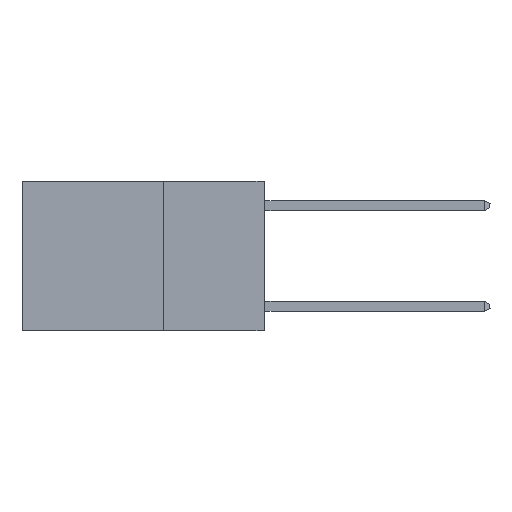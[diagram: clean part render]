
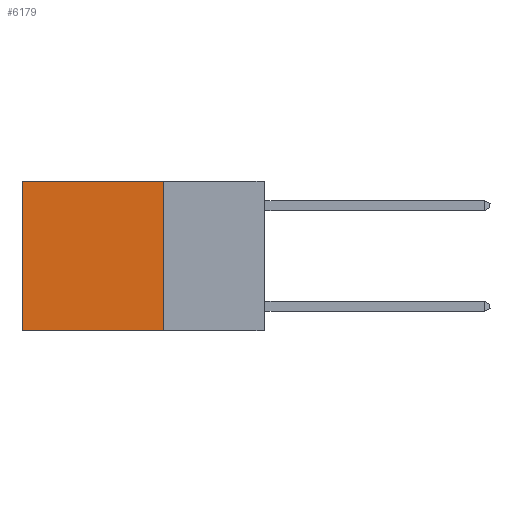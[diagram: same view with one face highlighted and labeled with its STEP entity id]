
A CAD part, left-side view. The second image highlights one B-rep face of the part: STEP entity #6179.
In plain terms, the highlighted planar face has unit normal (-1, 0, 0).
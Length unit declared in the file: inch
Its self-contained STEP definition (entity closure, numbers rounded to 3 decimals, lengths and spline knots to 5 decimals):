
#463 = VECTOR ( 'NONE', #7696, 39.37008 ) ;
#604 = DIRECTION ( 'NONE',  ( 0., 1., 0. ) ) ;
#834 = VECTOR ( 'NONE', #1040, 39.37008 ) ;
#1011 = EDGE_CURVE ( 'NONE', #14255, #8919, #1939, .T. ) ;
#1040 = DIRECTION ( 'NONE',  ( 0., 0., -1. ) ) ;
#1117 = CARTESIAN_POINT ( 'NONE',  ( 0.2625, 0.6, 0. ) ) ;
#1312 = VECTOR ( 'NONE', #604, 39.37008 ) ;
#1901 = LINE ( 'NONE', #1994, #1312 ) ;
#1939 = LINE ( 'NONE', #13079, #463 ) ;
#1994 = CARTESIAN_POINT ( 'NONE',  ( 0.2625, 0.25, -0.37 ) ) ;
#2526 = AXIS2_PLACEMENT_3D ( 'NONE', #12234, #15395, #13713 ) ;
#2606 = EDGE_CURVE ( 'NONE', #8919, #3448, #11747, .T. ) ;
#3366 = CARTESIAN_POINT ( 'NONE',  ( 0.2625, 0.25, -0.37 ) ) ;
#3448 = VERTEX_POINT ( 'NONE', #7010 ) ;
#3932 = CARTESIAN_POINT ( 'NONE',  ( 0.2625, 0.25, 0. ) ) ;
#5581 = ORIENTED_EDGE ( 'NONE', *, *, #1011, .T. ) ;
#6179 = ADVANCED_FACE ( 'NONE', ( #6669 ), #9768, .F. ) ;
#6669 = FACE_OUTER_BOUND ( 'NONE', #12794, .T. ) ;
#7010 = CARTESIAN_POINT ( 'NONE',  ( 0.2625, 0.6, -0.37 ) ) ;
#7696 = DIRECTION ( 'NONE',  ( 0., 1., 0. ) ) ;
#7801 = VECTOR ( 'NONE', #17135, 39.37008 ) ;
#8002 = LINE ( 'NONE', #9363, #834 ) ;
#8328 = EDGE_CURVE ( 'NONE', #10433, #3448, #1901, .T. ) ;
#8767 = CARTESIAN_POINT ( 'NONE',  ( 0.2625, 0.6, 0. ) ) ;
#8919 = VERTEX_POINT ( 'NONE', #1117 ) ;
#9363 = CARTESIAN_POINT ( 'NONE',  ( 0.2625, 0.25, 0. ) ) ;
#9768 = PLANE ( 'NONE',  #2526 ) ;
#9933 = ORIENTED_EDGE ( 'NONE', *, *, #13652, .F. ) ;
#10433 = VERTEX_POINT ( 'NONE', #3366 ) ;
#11747 = LINE ( 'NONE', #8767, #7801 ) ;
#12234 = CARTESIAN_POINT ( 'NONE',  ( 0.2625, 0.25, 0. ) ) ;
#12794 = EDGE_LOOP ( 'NONE', ( #17651, #15866, #9933, #5581 ) ) ;
#13079 = CARTESIAN_POINT ( 'NONE',  ( 0.2625, 0.25, 0. ) ) ;
#13652 = EDGE_CURVE ( 'NONE', #14255, #10433, #8002, .T. ) ;
#13713 = DIRECTION ( 'NONE',  ( 0., 0., -1. ) ) ;
#14255 = VERTEX_POINT ( 'NONE', #3932 ) ;
#15395 = DIRECTION ( 'NONE',  ( 1., 0., 0. ) ) ;
#15866 = ORIENTED_EDGE ( 'NONE', *, *, #8328, .F. ) ;
#17135 = DIRECTION ( 'NONE',  ( 0., 0., -1. ) ) ;
#17651 = ORIENTED_EDGE ( 'NONE', *, *, #2606, .T. ) ;
